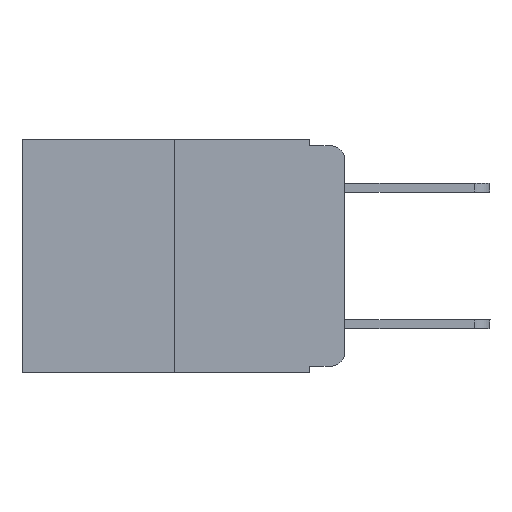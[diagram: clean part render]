
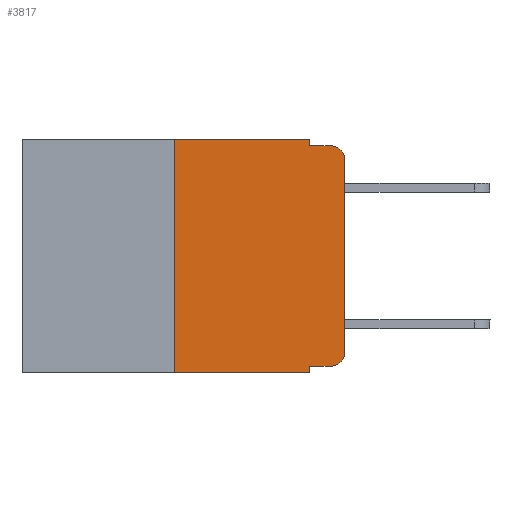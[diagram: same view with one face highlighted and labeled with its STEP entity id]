
A CAD part, left-side view. The second image highlights one B-rep face of the part: STEP entity #3817.
In plain terms, the highlighted planar face has unit normal (-1, 0, 0).
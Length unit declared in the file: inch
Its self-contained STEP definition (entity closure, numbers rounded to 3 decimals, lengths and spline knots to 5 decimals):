
#420 = ORIENTED_EDGE ( 'NONE', *, *, #2378, .F. ) ;
#648 = CARTESIAN_POINT ( 'NONE',  ( 0., 0.051, 0. ) ) ;
#689 = LINE ( 'NONE', #7614, #9250 ) ;
#715 = EDGE_CURVE ( 'NONE', #4769, #3654, #5934, .T. ) ;
#760 = CARTESIAN_POINT ( 'NONE',  ( 0., 0.25, 0. ) ) ;
#763 = VECTOR ( 'NONE', #7431, 39.37008 ) ;
#792 = EDGE_CURVE ( 'NONE', #8487, #4769, #6231, .T. ) ;
#816 = EDGE_CURVE ( 'NONE', #3654, #2905, #6381, .T. ) ;
#1190 = VECTOR ( 'NONE', #11979, 39.37008 ) ;
#1224 = ORIENTED_EDGE ( 'NONE', *, *, #816, .T. ) ;
#1797 = VECTOR ( 'NONE', #6825, 39.37008 ) ;
#2011 = CARTESIAN_POINT ( 'NONE',  ( 0., 0., 0. ) ) ;
#2016 = DIRECTION ( 'NONE',  ( 0., -1., 0. ) ) ;
#2035 = ORIENTED_EDGE ( 'NONE', *, *, #7363, .T. ) ;
#2097 = LINE ( 'NONE', #11641, #1797 ) ;
#2126 = ORIENTED_EDGE ( 'NONE', *, *, #6514, .F. ) ;
#2378 = EDGE_CURVE ( 'NONE', #4918, #10959, #6943, .T. ) ;
#2430 = DIRECTION ( 'NONE',  ( 0., 0., -1. ) ) ;
#2835 = CARTESIAN_POINT ( 'NONE',  ( 0., 0.02, -0.03 ) ) ;
#2905 = VERTEX_POINT ( 'NONE', #9145 ) ;
#2940 = VERTEX_POINT ( 'NONE', #5222 ) ;
#2972 = CARTESIAN_POINT ( 'NONE',  ( 0., 0.051, 0. ) ) ;
#3032 = VECTOR ( 'NONE', #7649, 39.37008 ) ;
#3122 = CARTESIAN_POINT ( 'NONE',  ( 0., 0.051, -0.333 ) ) ;
#3233 = AXIS2_PLACEMENT_3D ( 'NONE', #7704, #8528, #4790 ) ;
#3453 = AXIS2_PLACEMENT_3D ( 'NONE', #2835, #6794, #4756 ) ;
#3548 = CARTESIAN_POINT ( 'NONE',  ( 0., 0.02, -0.313 ) ) ;
#3654 = VERTEX_POINT ( 'NONE', #8323 ) ;
#3817 = ADVANCED_FACE ( 'NONE', ( #4640 ), #7743, .F. ) ;
#3966 = EDGE_CURVE ( 'NONE', #7893, #8487, #7489, .T. ) ;
#4111 = CARTESIAN_POINT ( 'NONE',  ( 0., 0.02, -0.333 ) ) ;
#4640 = FACE_OUTER_BOUND ( 'NONE', #10596, .T. ) ;
#4733 = CARTESIAN_POINT ( 'NONE',  ( 0., 0., -0.313 ) ) ;
#4756 = DIRECTION ( 'NONE',  ( 0., 0., -1. ) ) ;
#4769 = VERTEX_POINT ( 'NONE', #4733 ) ;
#4790 = DIRECTION ( 'NONE',  ( 0., 0., -1. ) ) ;
#4918 = VERTEX_POINT ( 'NONE', #2972 ) ;
#5222 = CARTESIAN_POINT ( 'NONE',  ( 0., 0.25, 0. ) ) ;
#5264 = CARTESIAN_POINT ( 'NONE',  ( 0., 0.051, 0. ) ) ;
#5326 = CARTESIAN_POINT ( 'NONE',  ( 0., 0.25, -0.343 ) ) ;
#5380 = DIRECTION ( 'NONE',  ( -1., 0., 0. ) ) ;
#5447 = ORIENTED_EDGE ( 'NONE', *, *, #9511, .F. ) ;
#5623 = VECTOR ( 'NONE', #11728, 39.37008 ) ;
#5826 = LINE ( 'NONE', #5264, #10788 ) ;
#5934 = LINE ( 'NONE', #2011, #5623 ) ;
#6231 = CIRCLE ( 'NONE', #12063, 0.02 ) ;
#6245 = DIRECTION ( 'NONE',  ( 0., 0., -1. ) ) ;
#6381 = CIRCLE ( 'NONE', #3453, 0.02 ) ;
#6514 = EDGE_CURVE ( 'NONE', #11363, #2940, #10833, .T. ) ;
#6587 = VERTEX_POINT ( 'NONE', #7600 ) ;
#6794 = DIRECTION ( 'NONE',  ( -1., 0., 0. ) ) ;
#6825 = DIRECTION ( 'NONE',  ( 0., -1., 0. ) ) ;
#6943 = LINE ( 'NONE', #648, #3032 ) ;
#7363 = EDGE_CURVE ( 'NONE', #11363, #6587, #12171, .T. ) ;
#7431 = DIRECTION ( 'NONE',  ( 0., 0., 1. ) ) ;
#7489 = LINE ( 'NONE', #3122, #10677 ) ;
#7600 = CARTESIAN_POINT ( 'NONE',  ( 0., 0.051, -0.343 ) ) ;
#7614 = CARTESIAN_POINT ( 'NONE',  ( 0., 0.473, 0. ) ) ;
#7649 = DIRECTION ( 'NONE',  ( 0., 0., -1. ) ) ;
#7704 = CARTESIAN_POINT ( 'NONE',  ( 0., 0.473, 0. ) ) ;
#7743 = PLANE ( 'NONE',  #3233 ) ;
#7893 = VERTEX_POINT ( 'NONE', #10925 ) ;
#8323 = CARTESIAN_POINT ( 'NONE',  ( 0., 0., -0.03 ) ) ;
#8487 = VERTEX_POINT ( 'NONE', #4111 ) ;
#8528 = DIRECTION ( 'NONE',  ( 1., 0., 0. ) ) ;
#9145 = CARTESIAN_POINT ( 'NONE',  ( 0., 0.02, -0.01 ) ) ;
#9153 = CARTESIAN_POINT ( 'NONE',  ( 0., 0.473, -0.343 ) ) ;
#9250 = VECTOR ( 'NONE', #2016, 39.37008 ) ;
#9261 = ORIENTED_EDGE ( 'NONE', *, *, #3966, .T. ) ;
#9511 = EDGE_CURVE ( 'NONE', #2940, #4918, #689, .T. ) ;
#9514 = ORIENTED_EDGE ( 'NONE', *, *, #12035, .F. ) ;
#10508 = EDGE_CURVE ( 'NONE', #7893, #6587, #5826, .T. ) ;
#10596 = EDGE_LOOP ( 'NONE', ( #10733, #1224, #9514, #420, #5447, #2126, #2035, #11050, #9261, #11797 ) ) ;
#10677 = VECTOR ( 'NONE', #11012, 39.37008 ) ;
#10733 = ORIENTED_EDGE ( 'NONE', *, *, #715, .T. ) ;
#10788 = VECTOR ( 'NONE', #2430, 39.37008 ) ;
#10833 = LINE ( 'NONE', #760, #763 ) ;
#10925 = CARTESIAN_POINT ( 'NONE',  ( 0., 0.051, -0.333 ) ) ;
#10959 = VERTEX_POINT ( 'NONE', #12447 ) ;
#11012 = DIRECTION ( 'NONE',  ( 0., -1., 0. ) ) ;
#11050 = ORIENTED_EDGE ( 'NONE', *, *, #10508, .F. ) ;
#11363 = VERTEX_POINT ( 'NONE', #5326 ) ;
#11641 = CARTESIAN_POINT ( 'NONE',  ( 0., 0.051, -0.01 ) ) ;
#11728 = DIRECTION ( 'NONE',  ( 0., 0., 1. ) ) ;
#11797 = ORIENTED_EDGE ( 'NONE', *, *, #792, .T. ) ;
#11979 = DIRECTION ( 'NONE',  ( 0., -1., 0. ) ) ;
#12035 = EDGE_CURVE ( 'NONE', #10959, #2905, #2097, .T. ) ;
#12063 = AXIS2_PLACEMENT_3D ( 'NONE', #3548, #5380, #6245 ) ;
#12171 = LINE ( 'NONE', #9153, #1190 ) ;
#12447 = CARTESIAN_POINT ( 'NONE',  ( 0., 0.051, -0.01 ) ) ;
